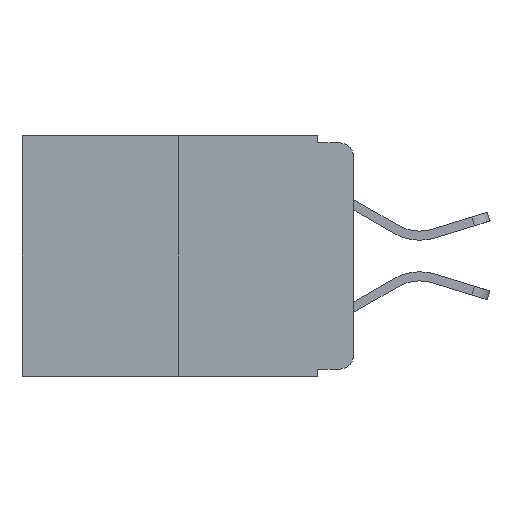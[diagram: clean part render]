
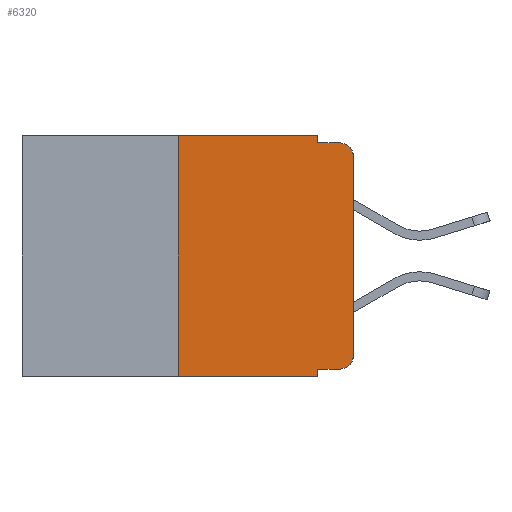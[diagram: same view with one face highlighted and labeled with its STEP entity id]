
A CAD part, left-side view. The second image highlights one B-rep face of the part: STEP entity #6320.
In plain terms, the highlighted planar face has unit normal (-1, 0, 0).
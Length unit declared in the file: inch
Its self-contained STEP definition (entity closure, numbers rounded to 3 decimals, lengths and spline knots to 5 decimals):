
#327 = CARTESIAN_POINT ( 'NONE',  ( 0., 0., -0.313 ) ) ;
#364 = EDGE_CURVE ( 'NONE', #1690, #694, #11922, .T. ) ;
#390 = VECTOR ( 'NONE', #22838, 39.37008 ) ;
#534 = ORIENTED_EDGE ( 'NONE', *, *, #22030, .F. ) ;
#618 = LINE ( 'NONE', #2728, #9812 ) ;
#694 = VERTEX_POINT ( 'NONE', #327 ) ;
#768 = LINE ( 'NONE', #2090, #14704 ) ;
#941 = VERTEX_POINT ( 'NONE', #15579 ) ;
#1003 = LINE ( 'NONE', #21094, #390 ) ;
#1131 = ORIENTED_EDGE ( 'NONE', *, *, #17024, .T. ) ;
#1437 = ORIENTED_EDGE ( 'NONE', *, *, #19277, .T. ) ;
#1497 = CARTESIAN_POINT ( 'NONE',  ( 0., 0.051, -0.333 ) ) ;
#1690 = VERTEX_POINT ( 'NONE', #14321 ) ;
#1933 = CARTESIAN_POINT ( 'NONE',  ( 0., 0.473, 0. ) ) ;
#2090 = CARTESIAN_POINT ( 'NONE',  ( 0., 0.25, 0. ) ) ;
#2182 = DIRECTION ( 'NONE',  ( 0., 0., -1. ) ) ;
#2519 = VERTEX_POINT ( 'NONE', #19888 ) ;
#2709 = LINE ( 'NONE', #21693, #11797 ) ;
#2728 = CARTESIAN_POINT ( 'NONE',  ( 0., 0.051, 0. ) ) ;
#2737 = EDGE_LOOP ( 'NONE', ( #1437, #20507, #21594, #13913, #23231, #534, #1131, #11433, #7792, #17242 ) ) ;
#2963 = VECTOR ( 'NONE', #8837, 39.37008 ) ;
#3544 = CARTESIAN_POINT ( 'NONE',  ( 0., 0.051, -0.343 ) ) ;
#3718 = EDGE_CURVE ( 'NONE', #5199, #21191, #13357, .T. ) ;
#4174 = CARTESIAN_POINT ( 'NONE',  ( 0., 0.473, 0. ) ) ;
#4367 = VECTOR ( 'NONE', #2182, 39.37008 ) ;
#5199 = VERTEX_POINT ( 'NONE', #17224 ) ;
#5319 = VERTEX_POINT ( 'NONE', #14129 ) ;
#6099 = VERTEX_POINT ( 'NONE', #19767 ) ;
#6197 = DIRECTION ( 'NONE',  ( 0., 0., -1. ) ) ;
#6320 = ADVANCED_FACE ( 'NONE', ( #16051 ), #22039, .F. ) ;
#7792 = ORIENTED_EDGE ( 'NONE', *, *, #10227, .T. ) ;
#8594 = VERTEX_POINT ( 'NONE', #10512 ) ;
#8837 = DIRECTION ( 'NONE',  ( 0., 0., 1. ) ) ;
#9732 = EDGE_CURVE ( 'NONE', #5319, #5199, #13440, .T. ) ;
#9775 = EDGE_CURVE ( 'NONE', #21191, #2519, #2709, .T. ) ;
#9812 = VECTOR ( 'NONE', #9947, 39.37008 ) ;
#9947 = DIRECTION ( 'NONE',  ( 0., 0., -1. ) ) ;
#10227 = EDGE_CURVE ( 'NONE', #941, #1690, #16465, .T. ) ;
#10280 = VERTEX_POINT ( 'NONE', #3544 ) ;
#10512 = CARTESIAN_POINT ( 'NONE',  ( 0., 0., -0.03 ) ) ;
#10671 = DIRECTION ( 'NONE',  ( 0., -1., 0. ) ) ;
#10990 = DIRECTION ( 'NONE',  ( -1., 0., 0. ) ) ;
#11087 = DIRECTION ( 'NONE',  ( 0., 0., 1. ) ) ;
#11201 = VECTOR ( 'NONE', #10671, 39.37008 ) ;
#11433 = ORIENTED_EDGE ( 'NONE', *, *, #18526, .F. ) ;
#11797 = VECTOR ( 'NONE', #19948, 39.37008 ) ;
#11922 = CIRCLE ( 'NONE', #17253, 0.02 ) ;
#12200 = EDGE_CURVE ( 'NONE', #8594, #2519, #16644, .T. ) ;
#12789 = DIRECTION ( 'NONE',  ( 0., -1., 0. ) ) ;
#13016 = CARTESIAN_POINT ( 'NONE',  ( 0., 0.051, 0. ) ) ;
#13357 = LINE ( 'NONE', #13016, #4367 ) ;
#13440 = LINE ( 'NONE', #1933, #22775 ) ;
#13913 = ORIENTED_EDGE ( 'NONE', *, *, #3718, .F. ) ;
#14129 = CARTESIAN_POINT ( 'NONE',  ( 0., 0.25, 0. ) ) ;
#14321 = CARTESIAN_POINT ( 'NONE',  ( 0., 0.02, -0.333 ) ) ;
#14704 = VECTOR ( 'NONE', #11087, 39.37008 ) ;
#15579 = CARTESIAN_POINT ( 'NONE',  ( 0., 0.051, -0.333 ) ) ;
#15925 = CARTESIAN_POINT ( 'NONE',  ( 0., 0., 0. ) ) ;
#16051 = FACE_OUTER_BOUND ( 'NONE', #2737, .T. ) ;
#16465 = LINE ( 'NONE', #1497, #11201 ) ;
#16644 = CIRCLE ( 'NONE', #16815, 0.02 ) ;
#16815 = AXIS2_PLACEMENT_3D ( 'NONE', #21525, #10990, #23265 ) ;
#16856 = DIRECTION ( 'NONE',  ( 1., 0., 0. ) ) ;
#17024 = EDGE_CURVE ( 'NONE', #6099, #10280, #1003, .T. ) ;
#17224 = CARTESIAN_POINT ( 'NONE',  ( 0., 0.051, 0. ) ) ;
#17242 = ORIENTED_EDGE ( 'NONE', *, *, #364, .T. ) ;
#17253 = AXIS2_PLACEMENT_3D ( 'NONE', #18707, #19140, #19034 ) ;
#17277 = LINE ( 'NONE', #15925, #2963 ) ;
#17915 = AXIS2_PLACEMENT_3D ( 'NONE', #4174, #16856, #6197 ) ;
#18526 = EDGE_CURVE ( 'NONE', #941, #10280, #618, .T. ) ;
#18707 = CARTESIAN_POINT ( 'NONE',  ( 0., 0.02, -0.313 ) ) ;
#19034 = DIRECTION ( 'NONE',  ( 0., 0., -1. ) ) ;
#19140 = DIRECTION ( 'NONE',  ( -1., 0., 0. ) ) ;
#19277 = EDGE_CURVE ( 'NONE', #694, #8594, #17277, .T. ) ;
#19767 = CARTESIAN_POINT ( 'NONE',  ( 0., 0.25, -0.343 ) ) ;
#19888 = CARTESIAN_POINT ( 'NONE',  ( 0., 0.02, -0.01 ) ) ;
#19948 = DIRECTION ( 'NONE',  ( 0., -1., 0. ) ) ;
#20507 = ORIENTED_EDGE ( 'NONE', *, *, #12200, .T. ) ;
#21094 = CARTESIAN_POINT ( 'NONE',  ( 0., 0.473, -0.343 ) ) ;
#21191 = VERTEX_POINT ( 'NONE', #21205 ) ;
#21205 = CARTESIAN_POINT ( 'NONE',  ( 0., 0.051, -0.01 ) ) ;
#21525 = CARTESIAN_POINT ( 'NONE',  ( 0., 0.02, -0.03 ) ) ;
#21594 = ORIENTED_EDGE ( 'NONE', *, *, #9775, .F. ) ;
#21693 = CARTESIAN_POINT ( 'NONE',  ( 0., 0.051, -0.01 ) ) ;
#22030 = EDGE_CURVE ( 'NONE', #6099, #5319, #768, .T. ) ;
#22039 = PLANE ( 'NONE',  #17915 ) ;
#22775 = VECTOR ( 'NONE', #12789, 39.37008 ) ;
#22838 = DIRECTION ( 'NONE',  ( 0., -1., 0. ) ) ;
#23231 = ORIENTED_EDGE ( 'NONE', *, *, #9732, .F. ) ;
#23265 = DIRECTION ( 'NONE',  ( 0., 0., -1. ) ) ;
